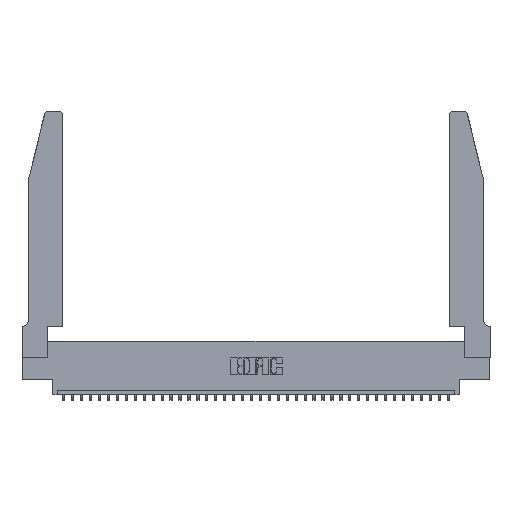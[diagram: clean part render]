
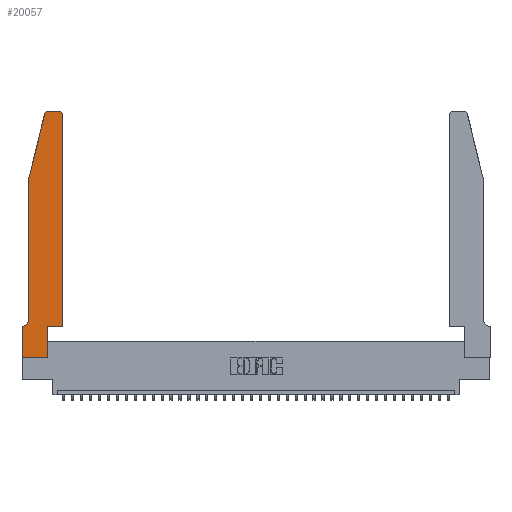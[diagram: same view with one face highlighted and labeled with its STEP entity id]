
A CAD part, top view. The second image highlights one B-rep face of the part: STEP entity #20057.
In plain terms, the highlighted planar face has unit normal (0, 0, 1).
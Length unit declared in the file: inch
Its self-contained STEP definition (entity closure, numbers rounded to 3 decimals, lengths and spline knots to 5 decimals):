
#562 = ORIENTED_EDGE ( 'NONE', *, *, #25471, .T. ) ;
#769 = CARTESIAN_POINT ( 'NONE',  ( 0., 0., 0.37 ) ) ;
#1290 = CARTESIAN_POINT ( 'NONE',  ( 0.4205, 2.72, 0.37 ) ) ;
#1300 = CIRCLE ( 'NONE', #23067, 0.07 ) ;
#1558 = CARTESIAN_POINT ( 'NONE',  ( 0.0755, 0.42, 0.37 ) ) ;
#1813 = ORIENTED_EDGE ( 'NONE', *, *, #27066, .T. ) ;
#2038 = CARTESIAN_POINT ( 'NONE',  ( 0.4505, 0.35, 0.37 ) ) ;
#2579 = VECTOR ( 'NONE', #9973, 39.37008 ) ;
#2828 = VECTOR ( 'NONE', #25344, 39.37008 ) ;
#4189 = EDGE_CURVE ( 'NONE', #29961, #23679, #9533, .T. ) ;
#4421 = CARTESIAN_POINT ( 'NONE',  ( 0.2865, 0.35, 0.37 ) ) ;
#5252 = VECTOR ( 'NONE', #16085, 39.37008 ) ;
#5603 = EDGE_CURVE ( 'NONE', #8153, #32607, #28601, .T. ) ;
#6272 = CARTESIAN_POINT ( 'NONE',  ( 0.284, 2.75, 0.37 ) ) ;
#6514 = ORIENTED_EDGE ( 'NONE', *, *, #14064, .T. ) ;
#7428 = ORIENTED_EDGE ( 'NONE', *, *, #35075, .T. ) ;
#7503 = LINE ( 'NONE', #27879, #11135 ) ;
#7542 = LINE ( 'NONE', #13135, #5252 ) ;
#8153 = VERTEX_POINT ( 'NONE', #24133 ) ;
#8659 = EDGE_LOOP ( 'NONE', ( #1813, #36727, #20722, #23744, #8684, #31567, #7428, #6514, #37502, #36084, #562, #10204 ) ) ;
#8684 = ORIENTED_EDGE ( 'NONE', *, *, #24876, .T. ) ;
#9024 = VECTOR ( 'NONE', #37434, 39.37008 ) ;
#9210 = CARTESIAN_POINT ( 'NONE',  ( 0.0755, 2., 0.37 ) ) ;
#9488 = VERTEX_POINT ( 'NONE', #19065 ) ;
#9491 = DIRECTION ( 'NONE',  ( 1., 0., 0. ) ) ;
#9533 = CIRCLE ( 'NONE', #31463, 0.03 ) ;
#9546 = AXIS2_PLACEMENT_3D ( 'NONE', #10224, #18533, #35950 ) ;
#9853 = LINE ( 'NONE', #9210, #31224 ) ;
#9973 = DIRECTION ( 'NONE',  ( 0., -1., 0. ) ) ;
#10204 = ORIENTED_EDGE ( 'NONE', *, *, #4189, .T. ) ;
#10224 = CARTESIAN_POINT ( 'NONE',  ( 0.284, 2.72, 0.37 ) ) ;
#11135 = VECTOR ( 'NONE', #36184, 39.37008 ) ;
#11695 = EDGE_CURVE ( 'NONE', #35516, #8153, #35471, .T. ) ;
#13109 = DIRECTION ( 'NONE',  ( 1., 0., 0. ) ) ;
#13135 = CARTESIAN_POINT ( 'NONE',  ( 0.0755, 0.35, 0.37 ) ) ;
#13789 = VERTEX_POINT ( 'NONE', #25303 ) ;
#14064 = EDGE_CURVE ( 'NONE', #23111, #35516, #36834, .T. ) ;
#15648 = DIRECTION ( 'NONE',  ( 0., 1., 0. ) ) ;
#15692 = CARTESIAN_POINT ( 'NONE',  ( 0., 0., 0.37 ) ) ;
#15933 = CARTESIAN_POINT ( 'NONE',  ( 0., 0.35, 0.37 ) ) ;
#16085 = DIRECTION ( 'NONE',  ( -1., 0., 0. ) ) ;
#16577 = CARTESIAN_POINT ( 'NONE',  ( 0.0755, 2., 0.37 ) ) ;
#18136 = VERTEX_POINT ( 'NONE', #1558 ) ;
#18190 = VECTOR ( 'NONE', #19098, 39.37008 ) ;
#18282 = DIRECTION ( 'NONE',  ( 0., -1., 0. ) ) ;
#18381 = CARTESIAN_POINT ( 'NONE',  ( 0.0055, 0.42, 0.37 ) ) ;
#18533 = DIRECTION ( 'NONE',  ( 0., 0., 1. ) ) ;
#19065 = CARTESIAN_POINT ( 'NONE',  ( 0.0055, 0.35, 0.37 ) ) ;
#19098 = DIRECTION ( 'NONE',  ( 0., 1., 0. ) ) ;
#19173 = FACE_OUTER_BOUND ( 'NONE', #8659, .T. ) ;
#19529 = AXIS2_PLACEMENT_3D ( 'NONE', #15933, #21524, #13109 ) ;
#20057 = ADVANCED_FACE ( 'NONE', ( #19173 ), #30792, .T. ) ;
#20230 = CARTESIAN_POINT ( 'NONE',  ( 0.25487, 2.72718, 0.37 ) ) ;
#20373 = CARTESIAN_POINT ( 'NONE',  ( 0., 0.35, 0.37 ) ) ;
#20722 = ORIENTED_EDGE ( 'NONE', *, *, #23367, .T. ) ;
#21350 = CIRCLE ( 'NONE', #9546, 0.03 ) ;
#21524 = DIRECTION ( 'NONE',  ( 0., 0., 1. ) ) ;
#21548 = CARTESIAN_POINT ( 'NONE',  ( 0., 0., 0.37 ) ) ;
#21833 = DIRECTION ( 'NONE',  ( 0., 0., 1. ) ) ;
#22777 = CARTESIAN_POINT ( 'NONE',  ( 0.4505, 0.35, 0.37 ) ) ;
#23067 = AXIS2_PLACEMENT_3D ( 'NONE', #18381, #24098, #27002 ) ;
#23111 = VERTEX_POINT ( 'NONE', #15692 ) ;
#23367 = EDGE_CURVE ( 'NONE', #35624, #13789, #29707, .T. ) ;
#23679 = VERTEX_POINT ( 'NONE', #36135 ) ;
#23744 = ORIENTED_EDGE ( 'NONE', *, *, #36411, .T. ) ;
#24098 = DIRECTION ( 'NONE',  ( 0., 0., -1. ) ) ;
#24133 = CARTESIAN_POINT ( 'NONE',  ( 0.2865, 0.35, 0.37 ) ) ;
#24876 = EDGE_CURVE ( 'NONE', #18136, #9488, #1300, .T. ) ;
#24892 = DIRECTION ( 'NONE',  ( 1., 0., 0. ) ) ;
#25303 = CARTESIAN_POINT ( 'NONE',  ( 0.0755, 2., 0.37 ) ) ;
#25344 = DIRECTION ( 'NONE',  ( -0.239, -0.971, 0. ) ) ;
#25471 = EDGE_CURVE ( 'NONE', #32607, #29961, #33172, .T. ) ;
#26730 = LINE ( 'NONE', #21548, #2579 ) ;
#27002 = DIRECTION ( 'NONE',  ( -1., 0., 0. ) ) ;
#27066 = EDGE_CURVE ( 'NONE', #23679, #36442, #7503, .T. ) ;
#27223 = CARTESIAN_POINT ( 'NONE',  ( 0.4505, 0.35, 0.37 ) ) ;
#27359 = VERTEX_POINT ( 'NONE', #20373 ) ;
#27835 = CARTESIAN_POINT ( 'NONE',  ( 0.2865, 0., 0.37 ) ) ;
#27879 = CARTESIAN_POINT ( 'NONE',  ( 0.2605, 2.75, 0.37 ) ) ;
#28601 = LINE ( 'NONE', #22777, #9024 ) ;
#29489 = VECTOR ( 'NONE', #15648, 39.37008 ) ;
#29707 = LINE ( 'NONE', #16577, #2828 ) ;
#29961 = VERTEX_POINT ( 'NONE', #34602 ) ;
#30792 = PLANE ( 'NONE',  #19529 ) ;
#30903 = EDGE_CURVE ( 'NONE', #36442, #35624, #21350, .T. ) ;
#31224 = VECTOR ( 'NONE', #18282, 39.37008 ) ;
#31463 = AXIS2_PLACEMENT_3D ( 'NONE', #1290, #21833, #24892 ) ;
#31567 = ORIENTED_EDGE ( 'NONE', *, *, #36662, .T. ) ;
#32607 = VERTEX_POINT ( 'NONE', #2038 ) ;
#33172 = LINE ( 'NONE', #27223, #29489 ) ;
#34602 = CARTESIAN_POINT ( 'NONE',  ( 0.4505, 2.72, 0.37 ) ) ;
#35075 = EDGE_CURVE ( 'NONE', #27359, #23111, #26730, .T. ) ;
#35471 = LINE ( 'NONE', #4421, #18190 ) ;
#35516 = VERTEX_POINT ( 'NONE', #27835 ) ;
#35624 = VERTEX_POINT ( 'NONE', #20230 ) ;
#35950 = DIRECTION ( 'NONE',  ( 1., 0., 0. ) ) ;
#36084 = ORIENTED_EDGE ( 'NONE', *, *, #5603, .T. ) ;
#36135 = CARTESIAN_POINT ( 'NONE',  ( 0.4205, 2.75, 0.37 ) ) ;
#36184 = DIRECTION ( 'NONE',  ( -1., 0., 0. ) ) ;
#36411 = EDGE_CURVE ( 'NONE', #13789, #18136, #9853, .T. ) ;
#36442 = VERTEX_POINT ( 'NONE', #6272 ) ;
#36662 = EDGE_CURVE ( 'NONE', #9488, #27359, #7542, .T. ) ;
#36727 = ORIENTED_EDGE ( 'NONE', *, *, #30903, .T. ) ;
#36834 = LINE ( 'NONE', #769, #37781 ) ;
#37434 = DIRECTION ( 'NONE',  ( 1., 0., 0. ) ) ;
#37502 = ORIENTED_EDGE ( 'NONE', *, *, #11695, .T. ) ;
#37781 = VECTOR ( 'NONE', #9491, 39.37008 ) ;
